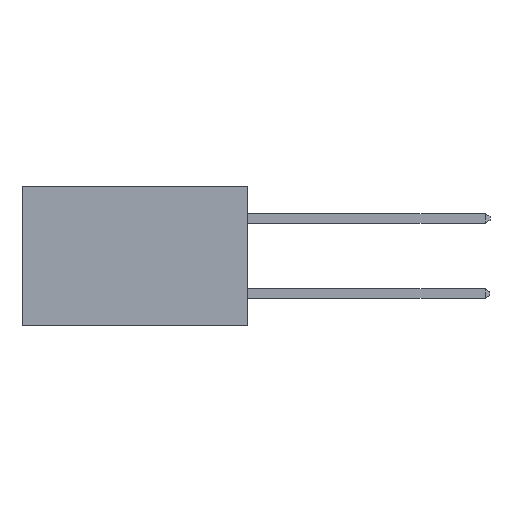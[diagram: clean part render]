
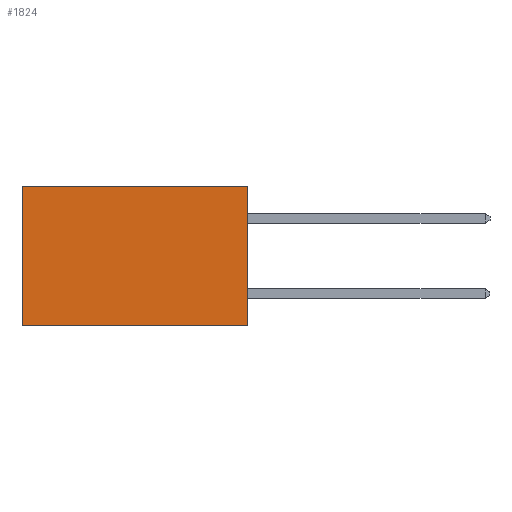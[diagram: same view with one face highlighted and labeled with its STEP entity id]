
A CAD part, left-side view. The second image highlights one B-rep face of the part: STEP entity #1824.
In plain terms, the highlighted planar face has unit normal (-1, 0, 0).
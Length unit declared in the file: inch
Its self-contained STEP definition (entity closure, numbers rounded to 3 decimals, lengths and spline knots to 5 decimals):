
#349 = CARTESIAN_POINT ( 'NONE',  ( 0.298, 0., 0. ) ) ;
#931 = EDGE_CURVE ( 'NONE', #1564, #6974, #1321, .T. ) ;
#951 = LINE ( 'NONE', #4611, #5835 ) ;
#1321 = LINE ( 'NONE', #2774, #8285 ) ;
#1468 = VERTEX_POINT ( 'NONE', #6925 ) ;
#1564 = VERTEX_POINT ( 'NONE', #5298 ) ;
#1824 = ADVANCED_FACE ( 'NONE', ( #5640 ), #9254, .F. ) ;
#2774 = CARTESIAN_POINT ( 'NONE',  ( 0.298, 0.6, 0. ) ) ;
#2889 = VECTOR ( 'NONE', #7284, 39.37008 ) ;
#2894 = LINE ( 'NONE', #7756, #9506 ) ;
#3925 = EDGE_CURVE ( 'NONE', #1468, #9380, #2894, .T. ) ;
#4065 = EDGE_CURVE ( 'NONE', #9380, #6974, #951, .T. ) ;
#4611 = CARTESIAN_POINT ( 'NONE',  ( 0.298, 0., -0.37 ) ) ;
#4787 = ORIENTED_EDGE ( 'NONE', *, *, #4065, .F. ) ;
#5154 = ORIENTED_EDGE ( 'NONE', *, *, #9362, .T. ) ;
#5186 = CARTESIAN_POINT ( 'NONE',  ( 0.298, 0.6, -0.37 ) ) ;
#5298 = CARTESIAN_POINT ( 'NONE',  ( 0.298, 0.6, 0. ) ) ;
#5360 = DIRECTION ( 'NONE',  ( 0., 0., -1. ) ) ;
#5640 = FACE_OUTER_BOUND ( 'NONE', #10031, .T. ) ;
#5835 = VECTOR ( 'NONE', #6393, 39.37008 ) ;
#6392 = ORIENTED_EDGE ( 'NONE', *, *, #3925, .F. ) ;
#6393 = DIRECTION ( 'NONE',  ( 0., 1., 0. ) ) ;
#6428 = CARTESIAN_POINT ( 'NONE',  ( 0.298, 0., -0.37 ) ) ;
#6920 = AXIS2_PLACEMENT_3D ( 'NONE', #9789, #7463, #9406 ) ;
#6925 = CARTESIAN_POINT ( 'NONE',  ( 0.298, 0., 0. ) ) ;
#6974 = VERTEX_POINT ( 'NONE', #5186 ) ;
#7229 = DIRECTION ( 'NONE',  ( 0., 0., -1. ) ) ;
#7284 = DIRECTION ( 'NONE',  ( 0., 1., 0. ) ) ;
#7463 = DIRECTION ( 'NONE',  ( 1., 0., 0. ) ) ;
#7756 = CARTESIAN_POINT ( 'NONE',  ( 0.298, 0., 0. ) ) ;
#8285 = VECTOR ( 'NONE', #7229, 39.37008 ) ;
#9254 = PLANE ( 'NONE',  #6920 ) ;
#9362 = EDGE_CURVE ( 'NONE', #1468, #1564, #9500, .T. ) ;
#9380 = VERTEX_POINT ( 'NONE', #6428 ) ;
#9406 = DIRECTION ( 'NONE',  ( 0., 0., -1. ) ) ;
#9500 = LINE ( 'NONE', #349, #2889 ) ;
#9506 = VECTOR ( 'NONE', #5360, 39.37008 ) ;
#9789 = CARTESIAN_POINT ( 'NONE',  ( 0.298, 0., 0. ) ) ;
#10031 = EDGE_LOOP ( 'NONE', ( #10428, #4787, #6392, #5154 ) ) ;
#10428 = ORIENTED_EDGE ( 'NONE', *, *, #931, .T. ) ;
